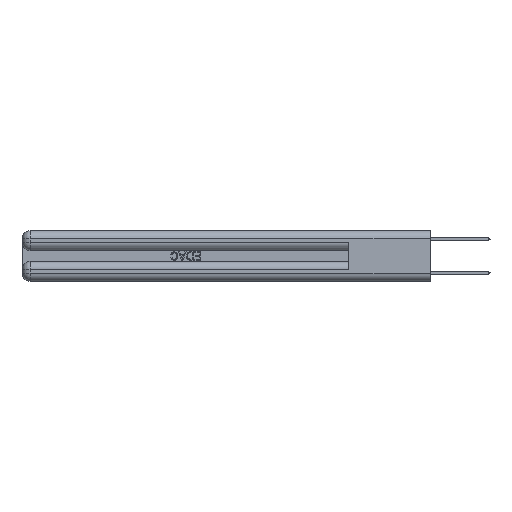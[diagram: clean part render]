
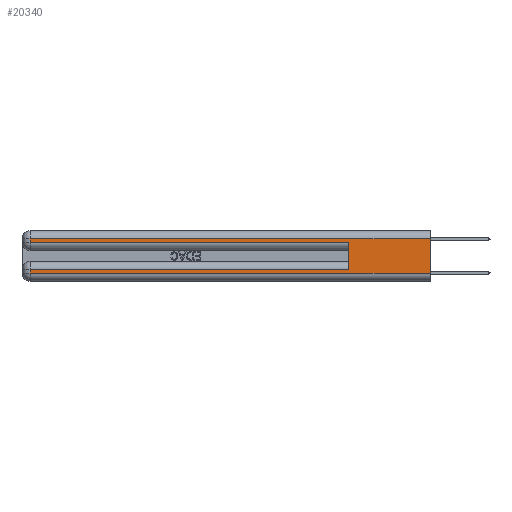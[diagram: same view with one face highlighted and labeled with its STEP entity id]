
A CAD part, left-side view. The second image highlights one B-rep face of the part: STEP entity #20340.
In plain terms, the highlighted planar face has unit normal (-1, 0, 0).
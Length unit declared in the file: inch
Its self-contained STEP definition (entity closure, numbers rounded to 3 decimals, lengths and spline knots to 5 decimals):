
#222 = ORIENTED_EDGE ( 'NONE', *, *, #27582, .F. ) ;
#1142 = VERTEX_POINT ( 'NONE', #33002 ) ;
#1182 = CARTESIAN_POINT ( 'NONE',  ( 0., 2.94, 0.31 ) ) ;
#1448 = CARTESIAN_POINT ( 'NONE',  ( 0., 0.6, 0.145 ) ) ;
#2651 = PLANE ( 'NONE',  #28994 ) ;
#2833 = CARTESIAN_POINT ( 'NONE',  ( 0., 0., 0.37 ) ) ;
#2844 = CARTESIAN_POINT ( 'NONE',  ( 0., 0., 0.285 ) ) ;
#2902 = CARTESIAN_POINT ( 'NONE',  ( 0., 2.94, 0.085 ) ) ;
#3024 = VECTOR ( 'NONE', #12176, 39.37008 ) ;
#3826 = VECTOR ( 'NONE', #6733, 39.37008 ) ;
#4827 = EDGE_CURVE ( 'NONE', #9955, #17785, #15792, .T. ) ;
#5161 = ORIENTED_EDGE ( 'NONE', *, *, #21943, .T. ) ;
#5411 = ORIENTED_EDGE ( 'NONE', *, *, #18479, .T. ) ;
#5420 = VERTEX_POINT ( 'NONE', #32706 ) ;
#5681 = VECTOR ( 'NONE', #22060, 39.37008 ) ;
#6733 = DIRECTION ( 'NONE',  ( 0., 1., 0. ) ) ;
#7424 = VERTEX_POINT ( 'NONE', #1182 ) ;
#8066 = CARTESIAN_POINT ( 'NONE',  ( 0., 0., 0.085 ) ) ;
#8436 = EDGE_CURVE ( 'NONE', #5420, #7424, #22689, .T. ) ;
#8504 = VECTOR ( 'NONE', #12992, 39.37008 ) ;
#8795 = ORIENTED_EDGE ( 'NONE', *, *, #21883, .T. ) ;
#8942 = CARTESIAN_POINT ( 'NONE',  ( 0., 0.6, 0.085 ) ) ;
#9955 = VERTEX_POINT ( 'NONE', #11798 ) ;
#10518 = VERTEX_POINT ( 'NONE', #25050 ) ;
#10520 = CARTESIAN_POINT ( 'NONE',  ( 0., 0., 0.06 ) ) ;
#11548 = ORIENTED_EDGE ( 'NONE', *, *, #4827, .T. ) ;
#11798 = CARTESIAN_POINT ( 'NONE',  ( 0., 2.94, 0.06 ) ) ;
#11832 = LINE ( 'NONE', #1448, #3024 ) ;
#12176 = DIRECTION ( 'NONE',  ( 0., 0., 1. ) ) ;
#12233 = VECTOR ( 'NONE', #33759, 39.37008 ) ;
#12992 = DIRECTION ( 'NONE',  ( 0., -1., 0. ) ) ;
#13053 = CARTESIAN_POINT ( 'NONE',  ( 0., 2.94, 0.37 ) ) ;
#13569 = DIRECTION ( 'NONE',  ( 1., 0., 0. ) ) ;
#14434 = ORIENTED_EDGE ( 'NONE', *, *, #25044, .T. ) ;
#14544 = VERTEX_POINT ( 'NONE', #8942 ) ;
#15507 = DIRECTION ( 'NONE',  ( 0., 0., -1. ) ) ;
#15792 = LINE ( 'NONE', #10520, #8504 ) ;
#16858 = CARTESIAN_POINT ( 'NONE',  ( 0., 0., 0.06 ) ) ;
#17243 = VECTOR ( 'NONE', #21267, 39.37008 ) ;
#17445 = CARTESIAN_POINT ( 'NONE',  ( 0., 0., 0.31 ) ) ;
#17472 = LINE ( 'NONE', #25337, #12233 ) ;
#17785 = VERTEX_POINT ( 'NONE', #16858 ) ;
#18138 = LINE ( 'NONE', #2844, #17243 ) ;
#18479 = EDGE_CURVE ( 'NONE', #7424, #10518, #30826, .T. ) ;
#19783 = CARTESIAN_POINT ( 'NONE',  ( 0., 2.94, 0.37 ) ) ;
#20340 = ADVANCED_FACE ( 'NONE', ( #30026 ), #2651, .F. ) ;
#21267 = DIRECTION ( 'NONE',  ( 0., -1., 0. ) ) ;
#21883 = EDGE_CURVE ( 'NONE', #10518, #1142, #18138, .T. ) ;
#21943 = EDGE_CURVE ( 'NONE', #29539, #9955, #29164, .T. ) ;
#22060 = DIRECTION ( 'NONE',  ( 0., 0., -1. ) ) ;
#22689 = LINE ( 'NONE', #17445, #3826 ) ;
#24026 = ORIENTED_EDGE ( 'NONE', *, *, #29575, .F. ) ;
#25044 = EDGE_CURVE ( 'NONE', #14544, #29539, #32077, .T. ) ;
#25050 = CARTESIAN_POINT ( 'NONE',  ( 0., 2.94, 0.285 ) ) ;
#25337 = CARTESIAN_POINT ( 'NONE',  ( 0., 0., 0.37 ) ) ;
#25541 = EDGE_LOOP ( 'NONE', ( #24026, #31542, #5411, #8795, #222, #14434, #5161, #11548 ) ) ;
#26193 = VECTOR ( 'NONE', #15507, 39.37008 ) ;
#26465 = VECTOR ( 'NONE', #26994, 39.37008 ) ;
#26994 = DIRECTION ( 'NONE',  ( 0., 1., 0. ) ) ;
#27582 = EDGE_CURVE ( 'NONE', #14544, #1142, #11832, .T. ) ;
#28994 = AXIS2_PLACEMENT_3D ( 'NONE', #2833, #13569, #32136 ) ;
#29164 = LINE ( 'NONE', #13053, #26193 ) ;
#29539 = VERTEX_POINT ( 'NONE', #2902 ) ;
#29575 = EDGE_CURVE ( 'NONE', #5420, #17785, #17472, .T. ) ;
#30026 = FACE_OUTER_BOUND ( 'NONE', #25541, .T. ) ;
#30826 = LINE ( 'NONE', #19783, #5681 ) ;
#31542 = ORIENTED_EDGE ( 'NONE', *, *, #8436, .T. ) ;
#32077 = LINE ( 'NONE', #8066, #26465 ) ;
#32136 = DIRECTION ( 'NONE',  ( 0., 0., -1. ) ) ;
#32706 = CARTESIAN_POINT ( 'NONE',  ( 0., 0., 0.31 ) ) ;
#33002 = CARTESIAN_POINT ( 'NONE',  ( 0., 0.6, 0.285 ) ) ;
#33759 = DIRECTION ( 'NONE',  ( 0., 0., -1. ) ) ;
